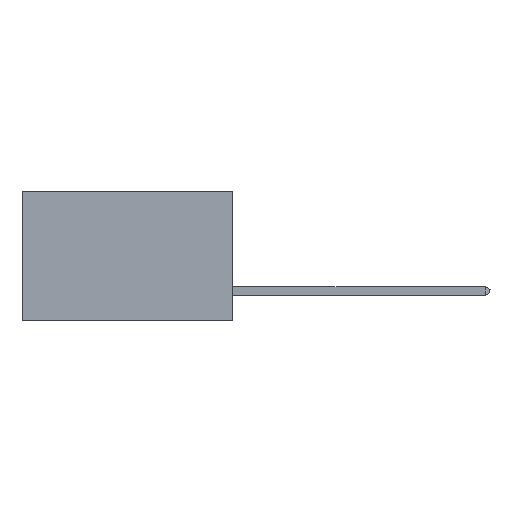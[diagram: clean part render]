
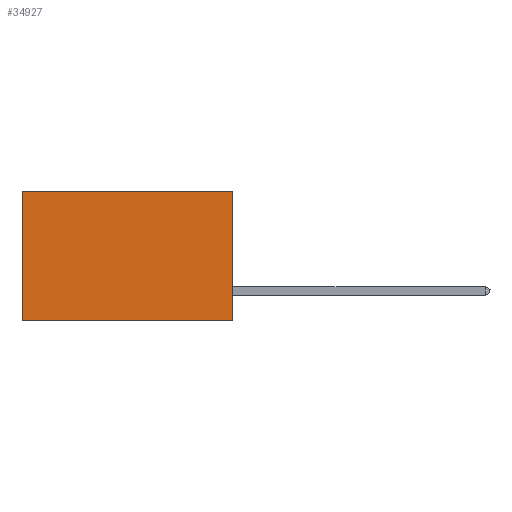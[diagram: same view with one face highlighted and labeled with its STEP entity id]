
A CAD part, left-side view. The second image highlights one B-rep face of the part: STEP entity #34927.
In plain terms, the highlighted planar face has unit normal (-1, 0, 0).
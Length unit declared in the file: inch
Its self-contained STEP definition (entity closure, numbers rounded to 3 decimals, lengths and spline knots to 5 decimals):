
#2184 = CARTESIAN_POINT ( 'NONE',  ( 0.2875, 0., 0. ) ) ;
#2361 = VERTEX_POINT ( 'NONE', #12211 ) ;
#2481 = EDGE_CURVE ( 'NONE', #26707, #3085, #17923, .T. ) ;
#2893 = LINE ( 'NONE', #7476, #31241 ) ;
#3085 = VERTEX_POINT ( 'NONE', #13718 ) ;
#4875 = DIRECTION ( 'NONE',  ( 0., 1., 0. ) ) ;
#5022 = DIRECTION ( 'NONE',  ( 0., 0., -1. ) ) ;
#6188 = EDGE_LOOP ( 'NONE', ( #20979, #13465, #30442, #32563 ) ) ;
#6905 = DIRECTION ( 'NONE',  ( 0., 1., 0. ) ) ;
#7476 = CARTESIAN_POINT ( 'NONE',  ( 0.2875, 0., -0.37 ) ) ;
#8366 = DIRECTION ( 'NONE',  ( 1., 0., 0. ) ) ;
#9500 = VERTEX_POINT ( 'NONE', #11026 ) ;
#9989 = LINE ( 'NONE', #21885, #25910 ) ;
#11026 = CARTESIAN_POINT ( 'NONE',  ( 0.2875, 0.6, 0. ) ) ;
#11932 = FACE_OUTER_BOUND ( 'NONE', #6188, .T. ) ;
#12211 = CARTESIAN_POINT ( 'NONE',  ( 0.2875, 0.6, -0.37 ) ) ;
#13465 = ORIENTED_EDGE ( 'NONE', *, *, #18011, .F. ) ;
#13718 = CARTESIAN_POINT ( 'NONE',  ( 0.2875, 0., -0.37 ) ) ;
#15393 = CARTESIAN_POINT ( 'NONE',  ( 0.2875, 0.6, 0. ) ) ;
#15453 = LINE ( 'NONE', #15393, #32755 ) ;
#17874 = DIRECTION ( 'NONE',  ( 0., 0., -1. ) ) ;
#17923 = LINE ( 'NONE', #2184, #34323 ) ;
#18011 = EDGE_CURVE ( 'NONE', #3085, #2361, #2893, .T. ) ;
#18056 = EDGE_CURVE ( 'NONE', #26707, #9500, #9989, .T. ) ;
#19242 = PLANE ( 'NONE',  #35287 ) ;
#20979 = ORIENTED_EDGE ( 'NONE', *, *, #23536, .T. ) ;
#21885 = CARTESIAN_POINT ( 'NONE',  ( 0.2875, 0., 0. ) ) ;
#22227 = DIRECTION ( 'NONE',  ( 0., 0., -1. ) ) ;
#23536 = EDGE_CURVE ( 'NONE', #9500, #2361, #15453, .T. ) ;
#25910 = VECTOR ( 'NONE', #6905, 39.37008 ) ;
#26707 = VERTEX_POINT ( 'NONE', #29552 ) ;
#29552 = CARTESIAN_POINT ( 'NONE',  ( 0.2875, 0., 0. ) ) ;
#30442 = ORIENTED_EDGE ( 'NONE', *, *, #2481, .F. ) ;
#31241 = VECTOR ( 'NONE', #4875, 39.37008 ) ;
#32563 = ORIENTED_EDGE ( 'NONE', *, *, #18056, .T. ) ;
#32755 = VECTOR ( 'NONE', #17874, 39.37008 ) ;
#34323 = VECTOR ( 'NONE', #22227, 39.37008 ) ;
#34927 = ADVANCED_FACE ( 'NONE', ( #11932 ), #19242, .F. ) ;
#35287 = AXIS2_PLACEMENT_3D ( 'NONE', #36513, #8366, #5022 ) ;
#36513 = CARTESIAN_POINT ( 'NONE',  ( 0.2875, 0., 0. ) ) ;
